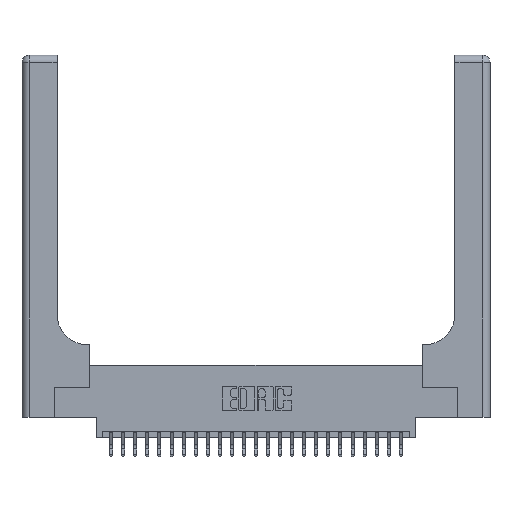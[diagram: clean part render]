
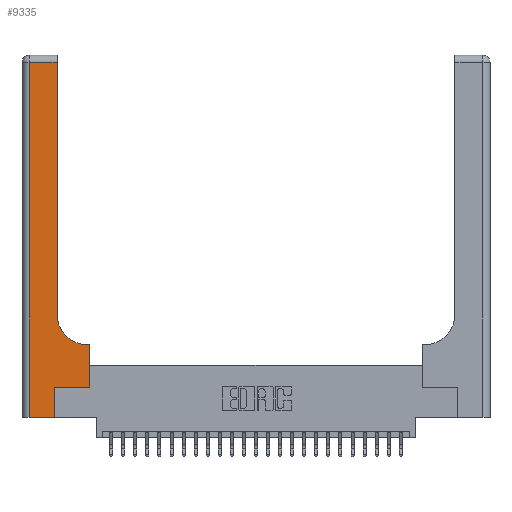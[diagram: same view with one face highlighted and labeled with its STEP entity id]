
A CAD part, top view. The second image highlights one B-rep face of the part: STEP entity #9335.
In plain terms, the highlighted planar face has unit normal (0, 0, 1).
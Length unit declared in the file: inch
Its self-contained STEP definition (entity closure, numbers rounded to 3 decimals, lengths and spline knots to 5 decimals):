
#117 = ORIENTED_EDGE ( 'NONE', *, *, #20023, .T. ) ;
#313 = LINE ( 'NONE', #14654, #16725 ) ;
#471 = VECTOR ( 'NONE', #12390, 39.37008 ) ;
#945 = VECTOR ( 'NONE', #13520, 39.37008 ) ;
#1137 = LINE ( 'NONE', #10318, #471 ) ;
#1278 = LINE ( 'NONE', #16468, #6444 ) ;
#2012 = AXIS2_PLACEMENT_3D ( 'NONE', #16690, #8343, #22986 ) ;
#2181 = DIRECTION ( 'NONE',  ( 1., 0., 0. ) ) ;
#2935 = ORIENTED_EDGE ( 'NONE', *, *, #7485, .T. ) ;
#3166 = VERTEX_POINT ( 'NONE', #11197 ) ;
#4042 = ORIENTED_EDGE ( 'NONE', *, *, #14969, .T. ) ;
#4643 = CARTESIAN_POINT ( 'NONE',  ( 0.5415, 0.85, 0.37 ) ) ;
#4842 = CARTESIAN_POINT ( 'NONE',  ( 0.269, 0.25, 0.37 ) ) ;
#5043 = ORIENTED_EDGE ( 'NONE', *, *, #18404, .T. ) ;
#6237 = CARTESIAN_POINT ( 'NONE',  ( 0., 2.94, 0.37 ) ) ;
#6444 = VECTOR ( 'NONE', #10280, 39.37008 ) ;
#6636 = CIRCLE ( 'NONE', #11760, 0.25 ) ;
#6730 = VERTEX_POINT ( 'NONE', #23283 ) ;
#6795 = LINE ( 'NONE', #19835, #945 ) ;
#6864 = DIRECTION ( 'NONE',  ( 1., 0., 0. ) ) ;
#7050 = DIRECTION ( 'NONE',  ( 1., 0., 0. ) ) ;
#7485 = EDGE_CURVE ( 'NONE', #13888, #6730, #23914, .T. ) ;
#7612 = CARTESIAN_POINT ( 'NONE',  ( 0.5585, 0.25, 0.37 ) ) ;
#8226 = EDGE_CURVE ( 'NONE', #25767, #13888, #6795, .T. ) ;
#8343 = DIRECTION ( 'NONE',  ( 0., 0., -1. ) ) ;
#8994 = CARTESIAN_POINT ( 'NONE',  ( 0.5415, 0.6, 0.37 ) ) ;
#9335 = ADVANCED_FACE ( 'NONE', ( #25116 ), #10403, .F. ) ;
#9430 = CARTESIAN_POINT ( 'NONE',  ( 0.2915, 2.94, 0.37 ) ) ;
#9541 = VERTEX_POINT ( 'NONE', #8994 ) ;
#9679 = ORIENTED_EDGE ( 'NONE', *, *, #8226, .T. ) ;
#10280 = DIRECTION ( 'NONE',  ( 0., 1., 0. ) ) ;
#10318 = CARTESIAN_POINT ( 'NONE',  ( 0.5585, 0.25, 0.37 ) ) ;
#10403 = PLANE ( 'NONE',  #2012 ) ;
#10476 = DIRECTION ( 'NONE',  ( 0., 1., 0. ) ) ;
#10516 = VERTEX_POINT ( 'NONE', #22564 ) ;
#11197 = CARTESIAN_POINT ( 'NONE',  ( 0.269, 0.25, 0.37 ) ) ;
#11760 = AXIS2_PLACEMENT_3D ( 'NONE', #4643, #19468, #6864 ) ;
#11961 = VERTEX_POINT ( 'NONE', #18146 ) ;
#12208 = LINE ( 'NONE', #4842, #22664 ) ;
#12390 = DIRECTION ( 'NONE',  ( 0., 1., 0. ) ) ;
#12856 = DIRECTION ( 'NONE',  ( -1., 0., 0. ) ) ;
#12927 = CARTESIAN_POINT ( 'NONE',  ( 0., 0., 0.37 ) ) ;
#13354 = EDGE_CURVE ( 'NONE', #23891, #11961, #1137, .T. ) ;
#13494 = ORIENTED_EDGE ( 'NONE', *, *, #15965, .T. ) ;
#13520 = DIRECTION ( 'NONE',  ( 0., -1., 0. ) ) ;
#13669 = VECTOR ( 'NONE', #18870, 39.37008 ) ;
#13888 = VERTEX_POINT ( 'NONE', #18587 ) ;
#14539 = LINE ( 'NONE', #27455, #15196 ) ;
#14654 = CARTESIAN_POINT ( 'NONE',  ( 0.269, 0., 0.37 ) ) ;
#14969 = EDGE_CURVE ( 'NONE', #3166, #23891, #12208, .T. ) ;
#15196 = VECTOR ( 'NONE', #12856, 39.37008 ) ;
#15965 = EDGE_CURVE ( 'NONE', #6730, #3166, #313, .T. ) ;
#16229 = ORIENTED_EDGE ( 'NONE', *, *, #20640, .T. ) ;
#16299 = VERTEX_POINT ( 'NONE', #9430 ) ;
#16468 = CARTESIAN_POINT ( 'NONE',  ( 0.2915, 3., 0.37 ) ) ;
#16641 = CARTESIAN_POINT ( 'NONE',  ( 0.06, 2.94, 0.37 ) ) ;
#16690 = CARTESIAN_POINT ( 'NONE',  ( 0., 3., 0.37 ) ) ;
#16725 = VECTOR ( 'NONE', #10476, 39.37008 ) ;
#18145 = ORIENTED_EDGE ( 'NONE', *, *, #23387, .T. ) ;
#18146 = CARTESIAN_POINT ( 'NONE',  ( 0.5585, 0.6, 0.37 ) ) ;
#18369 = VECTOR ( 'NONE', #2181, 39.37008 ) ;
#18404 = EDGE_CURVE ( 'NONE', #16299, #25767, #19241, .T. ) ;
#18587 = CARTESIAN_POINT ( 'NONE',  ( 0.06, 0., 0.37 ) ) ;
#18870 = DIRECTION ( 'NONE',  ( -1., 0., 0. ) ) ;
#19241 = LINE ( 'NONE', #6237, #13669 ) ;
#19399 = ORIENTED_EDGE ( 'NONE', *, *, #13354, .T. ) ;
#19468 = DIRECTION ( 'NONE',  ( 0., 0., -1. ) ) ;
#19835 = CARTESIAN_POINT ( 'NONE',  ( 0.06, 3., 0.37 ) ) ;
#20023 = EDGE_CURVE ( 'NONE', #9541, #10516, #6636, .T. ) ;
#20640 = EDGE_CURVE ( 'NONE', #11961, #9541, #14539, .T. ) ;
#22564 = CARTESIAN_POINT ( 'NONE',  ( 0.2915, 0.85, 0.37 ) ) ;
#22664 = VECTOR ( 'NONE', #7050, 39.37008 ) ;
#22986 = DIRECTION ( 'NONE',  ( -1., 0., 0. ) ) ;
#23283 = CARTESIAN_POINT ( 'NONE',  ( 0.269, 0., 0.37 ) ) ;
#23387 = EDGE_CURVE ( 'NONE', #10516, #16299, #1278, .T. ) ;
#23891 = VERTEX_POINT ( 'NONE', #7612 ) ;
#23914 = LINE ( 'NONE', #12927, #18369 ) ;
#24117 = EDGE_LOOP ( 'NONE', ( #18145, #5043, #9679, #2935, #13494, #4042, #19399, #16229, #117 ) ) ;
#25116 = FACE_OUTER_BOUND ( 'NONE', #24117, .T. ) ;
#25767 = VERTEX_POINT ( 'NONE', #16641 ) ;
#27455 = CARTESIAN_POINT ( 'NONE',  ( 0.2915, 0.6, 0.37 ) ) ;
